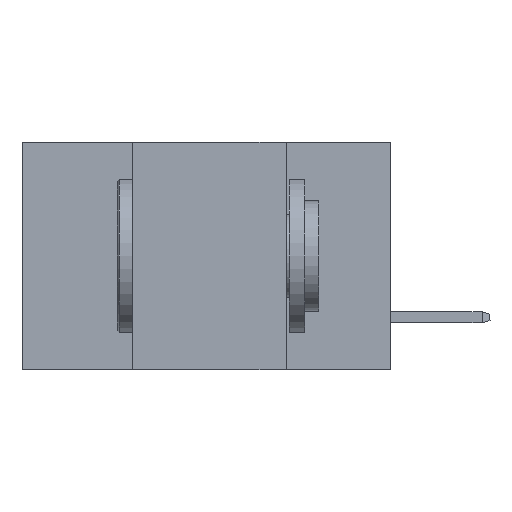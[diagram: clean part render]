
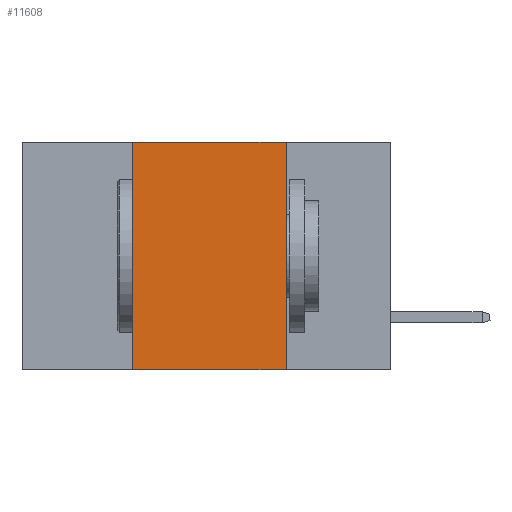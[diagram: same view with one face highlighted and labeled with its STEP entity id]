
A CAD part, left-side view. The second image highlights one B-rep face of the part: STEP entity #11608.
In plain terms, the highlighted planar face has unit normal (-1, 0, 0).
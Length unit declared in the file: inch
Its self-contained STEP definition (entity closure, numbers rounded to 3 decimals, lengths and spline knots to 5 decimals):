
#206 = VERTEX_POINT ( 'NONE', #6612 ) ;
#424 = CARTESIAN_POINT ( 'NONE',  ( 0., 0.17, 0. ) ) ;
#895 = PLANE ( 'NONE',  #7574 ) ;
#2446 = VECTOR ( 'NONE', #4583, 39.37008 ) ;
#2690 = EDGE_LOOP ( 'NONE', ( #12206, #7204, #12530, #5150 ) ) ;
#2773 = LINE ( 'NONE', #6550, #2446 ) ;
#2963 = CARTESIAN_POINT ( 'NONE',  ( 0., 0.6, 0. ) ) ;
#3495 = DIRECTION ( 'NONE',  ( 0., 0., -1. ) ) ;
#3563 = VECTOR ( 'NONE', #3495, 39.37008 ) ;
#3814 = CARTESIAN_POINT ( 'NONE',  ( 0., 0.42, 0. ) ) ;
#3976 = DIRECTION ( 'NONE',  ( 0., 0., -1. ) ) ;
#4160 = DIRECTION ( 'NONE',  ( 0., -1., 0. ) ) ;
#4300 = VERTEX_POINT ( 'NONE', #9156 ) ;
#4583 = DIRECTION ( 'NONE',  ( 0., -1., 0. ) ) ;
#4607 = EDGE_CURVE ( 'NONE', #4300, #206, #6251, .T. ) ;
#5083 = VERTEX_POINT ( 'NONE', #11223 ) ;
#5150 = ORIENTED_EDGE ( 'NONE', *, *, #10723, .T. ) ;
#6071 = FACE_OUTER_BOUND ( 'NONE', #2690, .T. ) ;
#6082 = LINE ( 'NONE', #11180, #8769 ) ;
#6251 = LINE ( 'NONE', #424, #3563 ) ;
#6477 = VECTOR ( 'NONE', #8849, 39.37008 ) ;
#6550 = CARTESIAN_POINT ( 'NONE',  ( 0., 0.6, -0.37 ) ) ;
#6612 = CARTESIAN_POINT ( 'NONE',  ( 0., 0.17, -0.37 ) ) ;
#6804 = LINE ( 'NONE', #3814, #6477 ) ;
#7204 = ORIENTED_EDGE ( 'NONE', *, *, #11129, .F. ) ;
#7574 = AXIS2_PLACEMENT_3D ( 'NONE', #2963, #10009, #3976 ) ;
#7810 = CARTESIAN_POINT ( 'NONE',  ( 0., 0.42, -0.37 ) ) ;
#7823 = EDGE_CURVE ( 'NONE', #12769, #5083, #6804, .T. ) ;
#8769 = VECTOR ( 'NONE', #4160, 39.37008 ) ;
#8849 = DIRECTION ( 'NONE',  ( 0., 0., 1. ) ) ;
#9156 = CARTESIAN_POINT ( 'NONE',  ( 0., 0.17, 0. ) ) ;
#10009 = DIRECTION ( 'NONE',  ( 1., 0., 0. ) ) ;
#10723 = EDGE_CURVE ( 'NONE', #12769, #206, #2773, .T. ) ;
#11129 = EDGE_CURVE ( 'NONE', #5083, #4300, #6082, .T. ) ;
#11180 = CARTESIAN_POINT ( 'NONE',  ( 0., 0.6, 0. ) ) ;
#11223 = CARTESIAN_POINT ( 'NONE',  ( 0., 0.42, 0. ) ) ;
#11608 = ADVANCED_FACE ( 'NONE', ( #6071 ), #895, .F. ) ;
#12206 = ORIENTED_EDGE ( 'NONE', *, *, #4607, .F. ) ;
#12530 = ORIENTED_EDGE ( 'NONE', *, *, #7823, .F. ) ;
#12769 = VERTEX_POINT ( 'NONE', #7810 ) ;
